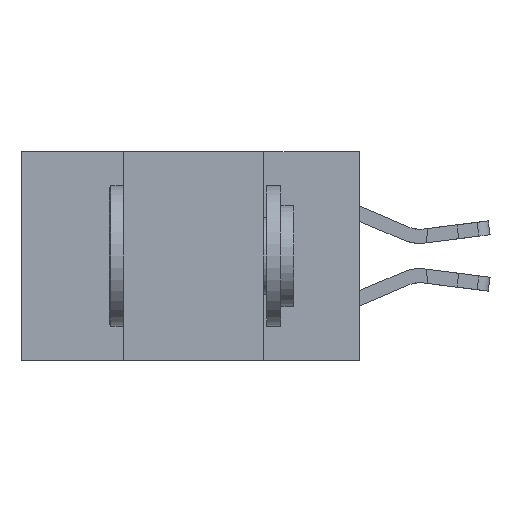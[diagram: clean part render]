
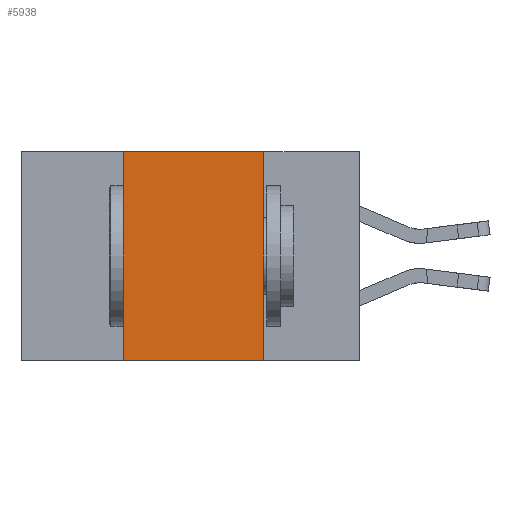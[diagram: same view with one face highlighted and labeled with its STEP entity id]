
A CAD part, left-side view. The second image highlights one B-rep face of the part: STEP entity #5938.
In plain terms, the highlighted planar face has unit normal (-1, 0, 0).
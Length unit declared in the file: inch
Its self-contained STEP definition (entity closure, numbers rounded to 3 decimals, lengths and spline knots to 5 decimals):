
#814 = DIRECTION ( 'NONE',  ( 0., -1., 0. ) ) ;
#1347 = DIRECTION ( 'NONE',  ( 0., 0., -1. ) ) ;
#1544 = CARTESIAN_POINT ( 'NONE',  ( 0., 0.17, 0. ) ) ;
#2935 = ORIENTED_EDGE ( 'NONE', *, *, #10988, .F. ) ;
#3928 = ORIENTED_EDGE ( 'NONE', *, *, #28122, .F. ) ;
#4603 = CARTESIAN_POINT ( 'NONE',  ( 0., 0.42, 0. ) ) ;
#5032 = VERTEX_POINT ( 'NONE', #24757 ) ;
#5938 = ADVANCED_FACE ( 'NONE', ( #24266 ), #30420, .F. ) ;
#7189 = EDGE_CURVE ( 'NONE', #23483, #9146, #7771, .T. ) ;
#7771 = LINE ( 'NONE', #10935, #27092 ) ;
#9036 = LINE ( 'NONE', #1544, #21262 ) ;
#9146 = VERTEX_POINT ( 'NONE', #30145 ) ;
#10639 = ORIENTED_EDGE ( 'NONE', *, *, #7189, .F. ) ;
#10935 = CARTESIAN_POINT ( 'NONE',  ( 0., 0.6, 0. ) ) ;
#10988 = EDGE_CURVE ( 'NONE', #9146, #28828, #9036, .T. ) ;
#11224 = CARTESIAN_POINT ( 'NONE',  ( 0., 0.6, 0. ) ) ;
#11683 = VECTOR ( 'NONE', #814, 39.37008 ) ;
#12012 = EDGE_CURVE ( 'NONE', #5032, #28828, #30070, .T. ) ;
#13167 = AXIS2_PLACEMENT_3D ( 'NONE', #11224, #16136, #1347 ) ;
#13881 = DIRECTION ( 'NONE',  ( 0., 0., -1. ) ) ;
#14531 = DIRECTION ( 'NONE',  ( 0., 0., 1. ) ) ;
#15658 = CARTESIAN_POINT ( 'NONE',  ( 0., 0.6, -0.37 ) ) ;
#16136 = DIRECTION ( 'NONE',  ( 1., 0., 0. ) ) ;
#21262 = VECTOR ( 'NONE', #13881, 39.37008 ) ;
#23064 = CARTESIAN_POINT ( 'NONE',  ( 0., 0.42, 0. ) ) ;
#23443 = EDGE_LOOP ( 'NONE', ( #2935, #10639, #3928, #24056 ) ) ;
#23483 = VERTEX_POINT ( 'NONE', #23064 ) ;
#24056 = ORIENTED_EDGE ( 'NONE', *, *, #12012, .T. ) ;
#24266 = FACE_OUTER_BOUND ( 'NONE', #23443, .T. ) ;
#24362 = CARTESIAN_POINT ( 'NONE',  ( 0., 0.17, -0.37 ) ) ;
#24543 = VECTOR ( 'NONE', #14531, 39.37008 ) ;
#24757 = CARTESIAN_POINT ( 'NONE',  ( 0., 0.42, -0.37 ) ) ;
#25449 = DIRECTION ( 'NONE',  ( 0., -1., 0. ) ) ;
#27092 = VECTOR ( 'NONE', #25449, 39.37008 ) ;
#28122 = EDGE_CURVE ( 'NONE', #5032, #23483, #30758, .T. ) ;
#28828 = VERTEX_POINT ( 'NONE', #24362 ) ;
#30070 = LINE ( 'NONE', #15658, #11683 ) ;
#30145 = CARTESIAN_POINT ( 'NONE',  ( 0., 0.17, 0. ) ) ;
#30420 = PLANE ( 'NONE',  #13167 ) ;
#30758 = LINE ( 'NONE', #4603, #24543 ) ;
